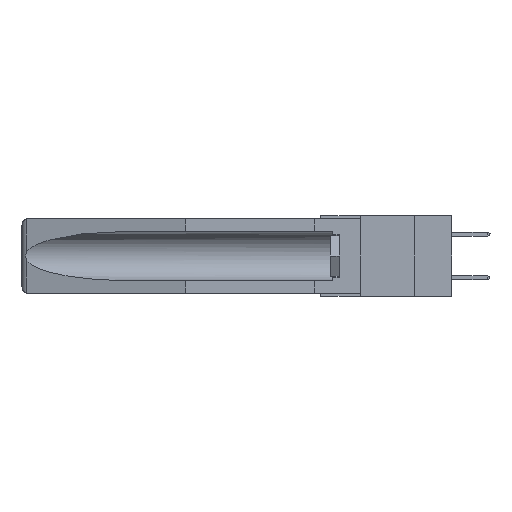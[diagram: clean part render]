
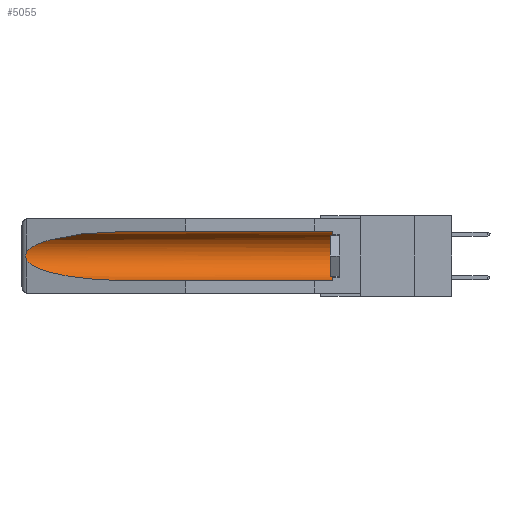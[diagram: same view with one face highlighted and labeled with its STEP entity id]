
A CAD part, left-side view. The second image highlights one B-rep face of the part: STEP entity #5055.
In plain terms, the highlighted cylindrical face has radius 2.857 mm (diameter 5.715 mm), a partial arc.
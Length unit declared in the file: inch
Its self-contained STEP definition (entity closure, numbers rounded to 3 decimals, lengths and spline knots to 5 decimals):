
#514 = DIRECTION ( 'NONE',  ( 0., 1., 0. ) ) ;
#705 = CARTESIAN_POINT ( 'NONE',  ( 0.26655, 1.53094, -0.18657 ) ) ;
#1682 = LINE ( 'NONE', #6666, #16443 ) ;
#2469 = LINE ( 'NONE', #6488, #11101 ) ;
#3142 = VERTEX_POINT ( 'NONE', #7355 ) ;
#3431 = CARTESIAN_POINT ( 'NONE',  ( 0.2675, 1.53308, -0.16763 ) ) ;
#3760 = CARTESIAN_POINT ( 'NONE',  ( 0.26654, 1.53092, -0.15636 ) ) ;
#4588 = VERTEX_POINT ( 'NONE', #33602 ) ;
#4691 = CARTESIAN_POINT ( 'NONE',  ( 0.155, 1.07973, -0.059 ) ) ;
#4978 = CYLINDRICAL_SURFACE ( 'NONE', #21760, 0.1125 ) ;
#5055 = ADVANCED_FACE ( 'NONE', ( #29220 ), #4978, .F. ) ;
#5474 = VERTEX_POINT ( 'NONE', #20263 ) ;
#5501 = B_SPLINE_CURVE_WITH_KNOTS ( 'NONE', 3,
 ( #16374, #27066, #3760, #29587, #3431, #8588, #13843, #705, #14070, #8823 ),
 .UNSPECIFIED., .F., .F.,
 ( 4, 2, 2, 2, 4 ),
 ( 0., 0.00029, 0.00058, 0.00087, 0.00117 ),
 .UNSPECIFIED. ) ;
#5793 = EDGE_CURVE ( 'NONE', #3142, #19411, #1682, .T. ) ;
#6025 = EDGE_LOOP ( 'NONE', ( #33242, #11592, #12871, #18423, #12346, #26664 ) ) ;
#6189 = EDGE_CURVE ( 'NONE', #26292, #30721, #2469, .T. ) ;
#6488 = CARTESIAN_POINT ( 'NONE',  ( 0.155, -0.30754, -0.059 ) ) ;
#6666 = CARTESIAN_POINT ( 'NONE',  ( 0.155, -0.30754, -0.284 ) ) ;
#7328 = CARTESIAN_POINT ( 'NONE',  ( 0.21114, 1.30732, -0.059 ) ) ;
#7355 = CARTESIAN_POINT ( 'NONE',  ( 0.155, 0.126, -0.284 ) ) ;
#8588 = CARTESIAN_POINT ( 'NONE',  ( 0.2675, 1.53308, -0.17534 ) ) ;
#8735 = DIRECTION ( 'NONE',  ( 0., 0., 1. ) ) ;
#8823 = CARTESIAN_POINT ( 'NONE',  ( 0.26537, 1.52718, -0.19328 ) ) ;
#10901 = CARTESIAN_POINT ( 'NONE',  ( 0.155, 0.126, -0.1715 ) ) ;
#11101 = VECTOR ( 'NONE', #24747, 39.37008 ) ;
#11592 = ORIENTED_EDGE ( 'NONE', *, *, #17724, .T. ) ;
#11662 = EDGE_CURVE ( 'NONE', #3142, #26292, #21701, .T. ) ;
#12346 = ORIENTED_EDGE ( 'NONE', *, *, #11662, .T. ) ;
#12871 = ORIENTED_EDGE ( 'NONE', *, *, #23116, .T. ) ;
#13156 = CARTESIAN_POINT ( 'NONE',  ( 0.26537, 1.52718, -0.14972 ) ) ;
#13843 = CARTESIAN_POINT ( 'NONE',  ( 0.2673, 1.53269, -0.17917 ) ) ;
#14070 = CARTESIAN_POINT ( 'NONE',  ( 0.26597, 1.5296, -0.19026 ) ) ;
#16374 = CARTESIAN_POINT ( 'NONE',  ( 0.26537, 1.52718, -0.14972 ) ) ;
#16443 = VECTOR ( 'NONE', #21555, 39.37008 ) ;
#17020 = CARTESIAN_POINT ( 'NONE',  ( 0.155, 1.07973, -0.284 ) ) ;
#17724 = EDGE_CURVE ( 'NONE', #5474, #4588, #5501, .T. ) ;
#18423 = ORIENTED_EDGE ( 'NONE', *, *, #5793, .F. ) ;
#19237 = CARTESIAN_POINT ( 'NONE',  ( 0.155, 1.07973, -0.284 ) ) ;
#19411 = VERTEX_POINT ( 'NONE', #19237 ) ;
#20263 = CARTESIAN_POINT ( 'NONE',  ( 0.26537, 1.52718, -0.14972 ) ) ;
#20532 = CARTESIAN_POINT ( 'NONE',  ( 0.25451, 1.48313, -0.09465 ) ) ;
#21555 = DIRECTION ( 'NONE',  ( 0., 1., 0. ) ) ;
#21698 =( BOUNDED_CURVE ( )  B_SPLINE_CURVE ( 3, ( #4691, #7328, #20532, #13156 ),
 .UNSPECIFIED., .F., .F. ) 
 B_SPLINE_CURVE_WITH_KNOTS ( ( 4, 4 ),
 ( 4.71239, 6.08839 ),
 .UNSPECIFIED. ) 
 CURVE ( )  GEOMETRIC_REPRESENTATION_ITEM ( )  RATIONAL_B_SPLINE_CURVE ( ( 1., 0.848, 0.848, 1. ) ) 
 REPRESENTATION_ITEM ( '' )  );
#21701 = CIRCLE ( 'NONE', #21721, 0.1125 ) ;
#21721 = AXIS2_PLACEMENT_3D ( 'NONE', #10901, #29243, #26949 ) ;
#21760 = AXIS2_PLACEMENT_3D ( 'NONE', #32256, #514, #8735 ) ;
#21815 = EDGE_CURVE ( 'NONE', #30721, #5474, #21698, .T. ) ;
#22411 = CARTESIAN_POINT ( 'NONE',  ( 0.25451, 1.48313, -0.24835 ) ) ;
#23116 = EDGE_CURVE ( 'NONE', #4588, #19411, #33478, .T. ) ;
#24747 = DIRECTION ( 'NONE',  ( 0., 1., 0. ) ) ;
#26292 = VERTEX_POINT ( 'NONE', #33181 ) ;
#26664 = ORIENTED_EDGE ( 'NONE', *, *, #6189, .T. ) ;
#26949 = DIRECTION ( 'NONE',  ( 0., 0., 1. ) ) ;
#27066 = CARTESIAN_POINT ( 'NONE',  ( 0.26597, 1.52961, -0.15275 ) ) ;
#29220 = FACE_OUTER_BOUND ( 'NONE', #6025, .T. ) ;
#29243 = DIRECTION ( 'NONE',  ( 0., -1., 0. ) ) ;
#29587 = CARTESIAN_POINT ( 'NONE',  ( 0.2673, 1.5327, -0.16383 ) ) ;
#30721 = VERTEX_POINT ( 'NONE', #31263 ) ;
#31263 = CARTESIAN_POINT ( 'NONE',  ( 0.155, 1.07973, -0.059 ) ) ;
#32256 = CARTESIAN_POINT ( 'NONE',  ( 0.155, -0.30754, -0.1715 ) ) ;
#32631 = CARTESIAN_POINT ( 'NONE',  ( 0.21114, 1.30732, -0.284 ) ) ;
#32854 = CARTESIAN_POINT ( 'NONE',  ( 0.26537, 1.52718, -0.19328 ) ) ;
#33181 = CARTESIAN_POINT ( 'NONE',  ( 0.155, 0.126, -0.059 ) ) ;
#33242 = ORIENTED_EDGE ( 'NONE', *, *, #21815, .T. ) ;
#33478 =( BOUNDED_CURVE ( )  B_SPLINE_CURVE ( 3, ( #32854, #22411, #32631, #17020 ),
 .UNSPECIFIED., .F., .F. ) 
 B_SPLINE_CURVE_WITH_KNOTS ( ( 4, 4 ),
 ( 0.1948, 1.5708 ),
 .UNSPECIFIED. ) 
 CURVE ( )  GEOMETRIC_REPRESENTATION_ITEM ( )  RATIONAL_B_SPLINE_CURVE ( ( 1., 0.848, 0.848, 1. ) ) 
 REPRESENTATION_ITEM ( '' )  );
#33602 = CARTESIAN_POINT ( 'NONE',  ( 0.26537, 1.52718, -0.19328 ) ) ;
